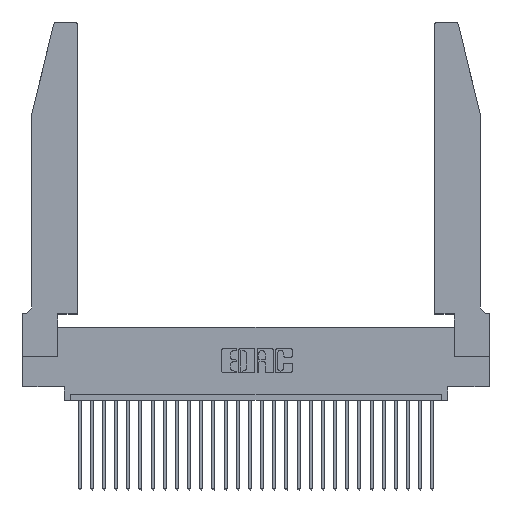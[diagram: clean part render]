
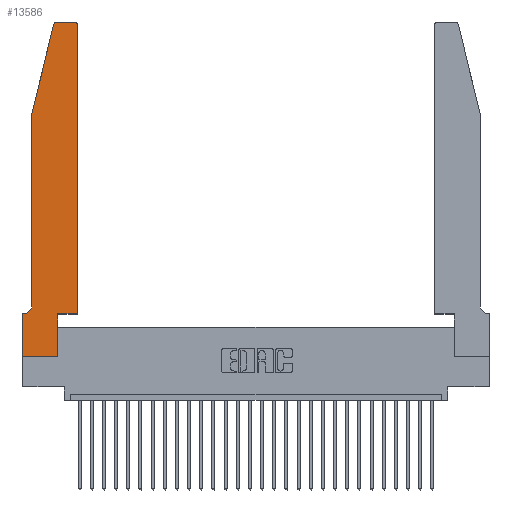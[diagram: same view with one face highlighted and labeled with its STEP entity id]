
A CAD part, top view. The second image highlights one B-rep face of the part: STEP entity #13586.
In plain terms, the highlighted planar face has unit normal (0, 0, 1).
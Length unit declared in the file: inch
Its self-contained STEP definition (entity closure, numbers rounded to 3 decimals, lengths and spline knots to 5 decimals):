
#89 = EDGE_LOOP ( 'NONE', ( #27496, #6674, #12539, #21687, #1411, #23947, #21259, #15491, #24205, #21631, #15594, #18094 ) ) ;
#479 = CIRCLE ( 'NONE', #1460, 0.03 ) ;
#762 = CIRCLE ( 'NONE', #11678, 0.03 ) ;
#1195 = CARTESIAN_POINT ( 'NONE',  ( 0.0755, 0.35, 0.37 ) ) ;
#1411 = ORIENTED_EDGE ( 'NONE', *, *, #18898, .T. ) ;
#1460 = AXIS2_PLACEMENT_3D ( 'NONE', #28780, #13288, #13474 ) ;
#1652 = VECTOR ( 'NONE', #7320, 39.37008 ) ;
#1716 = LINE ( 'NONE', #27912, #24635 ) ;
#1842 = EDGE_CURVE ( 'NONE', #8224, #24900, #9375, .T. ) ;
#1950 = EDGE_CURVE ( 'NONE', #25447, #23600, #9041, .T. ) ;
#1975 = EDGE_CURVE ( 'NONE', #24900, #28702, #24199, .T. ) ;
#2297 = DIRECTION ( 'NONE',  ( 0., -1., 0. ) ) ;
#2299 = CARTESIAN_POINT ( 'NONE',  ( 0.4505, 0.35, 0.37 ) ) ;
#2586 = CARTESIAN_POINT ( 'NONE',  ( 0.4205, 2.72, 0.37 ) ) ;
#2910 = CARTESIAN_POINT ( 'NONE',  ( 0.4505, 0.35, 0.37 ) ) ;
#3009 = VECTOR ( 'NONE', #19005, 39.37008 ) ;
#3139 = CARTESIAN_POINT ( 'NONE',  ( 0., 0.35, 0.37 ) ) ;
#3147 = DIRECTION ( 'NONE',  ( 0., 1., 0. ) ) ;
#3541 = CARTESIAN_POINT ( 'NONE',  ( 0., 0.35, 0.37 ) ) ;
#3924 = CARTESIAN_POINT ( 'NONE',  ( 0., 0., 0.37 ) ) ;
#5821 = CARTESIAN_POINT ( 'NONE',  ( 0.2865, 0.35, 0.37 ) ) ;
#5975 = CARTESIAN_POINT ( 'NONE',  ( 0.4505, 2.72, 0.37 ) ) ;
#6007 = VECTOR ( 'NONE', #9335, 39.37008 ) ;
#6084 = LINE ( 'NONE', #1195, #14186 ) ;
#6195 = DIRECTION ( 'NONE',  ( 1., 0., 0. ) ) ;
#6674 = ORIENTED_EDGE ( 'NONE', *, *, #12364, .T. ) ;
#7122 = AXIS2_PLACEMENT_3D ( 'NONE', #3139, #7982, #6195 ) ;
#7320 = DIRECTION ( 'NONE',  ( 0., -1., 0. ) ) ;
#7804 = CARTESIAN_POINT ( 'NONE',  ( 0.2605, 2.75, 0.37 ) ) ;
#7982 = DIRECTION ( 'NONE',  ( 0., 0., 1. ) ) ;
#8064 = EDGE_CURVE ( 'NONE', #21774, #8224, #6084, .T. ) ;
#8224 = VERTEX_POINT ( 'NONE', #3541 ) ;
#8480 = PLANE ( 'NONE',  #7122 ) ;
#9041 = LINE ( 'NONE', #27395, #9745 ) ;
#9335 = DIRECTION ( 'NONE',  ( 1., 0., 0. ) ) ;
#9375 = LINE ( 'NONE', #25190, #1652 ) ;
#9668 = DIRECTION ( 'NONE',  ( 1., 0., 0. ) ) ;
#9745 = VECTOR ( 'NONE', #2297, 39.37008 ) ;
#9904 = CARTESIAN_POINT ( 'NONE',  ( 0.0055, 0.35, 0.37 ) ) ;
#10312 = CARTESIAN_POINT ( 'NONE',  ( 0.25487, 2.72718, 0.37 ) ) ;
#10674 = FACE_OUTER_BOUND ( 'NONE', #89, .T. ) ;
#11245 = EDGE_CURVE ( 'NONE', #26189, #24770, #24901, .T. ) ;
#11678 = AXIS2_PLACEMENT_3D ( 'NONE', #2586, #13980, #9668 ) ;
#11720 = VERTEX_POINT ( 'NONE', #21074 ) ;
#11936 = DIRECTION ( 'NONE',  ( -1., 0., 0. ) ) ;
#12044 = CARTESIAN_POINT ( 'NONE',  ( 0.0055, 0.42, 0.37 ) ) ;
#12217 = VECTOR ( 'NONE', #22339, 39.37008 ) ;
#12364 = EDGE_CURVE ( 'NONE', #28287, #26040, #479, .T. ) ;
#12539 = ORIENTED_EDGE ( 'NONE', *, *, #19051, .T. ) ;
#13288 = DIRECTION ( 'NONE',  ( 0., 0., 1. ) ) ;
#13474 = DIRECTION ( 'NONE',  ( 1., 0., 0. ) ) ;
#13586 = ADVANCED_FACE ( 'NONE', ( #10674 ), #8480, .T. ) ;
#13980 = DIRECTION ( 'NONE',  ( 0., 0., 1. ) ) ;
#14186 = VECTOR ( 'NONE', #23722, 39.37008 ) ;
#14214 = AXIS2_PLACEMENT_3D ( 'NONE', #12044, #18595, #11936 ) ;
#14580 = DIRECTION ( 'NONE',  ( -0.239, -0.971, 0. ) ) ;
#14639 = EDGE_CURVE ( 'NONE', #24770, #25702, #762, .T. ) ;
#15466 = CIRCLE ( 'NONE', #14214, 0.07 ) ;
#15491 = ORIENTED_EDGE ( 'NONE', *, *, #1975, .T. ) ;
#15594 = ORIENTED_EDGE ( 'NONE', *, *, #11245, .T. ) ;
#16029 = CARTESIAN_POINT ( 'NONE',  ( 0.4205, 2.75, 0.37 ) ) ;
#18094 = ORIENTED_EDGE ( 'NONE', *, *, #14639, .T. ) ;
#18595 = DIRECTION ( 'NONE',  ( 0., 0., -1. ) ) ;
#18861 = VECTOR ( 'NONE', #3147, 39.37008 ) ;
#18898 = EDGE_CURVE ( 'NONE', #23600, #21774, #15466, .T. ) ;
#19005 = DIRECTION ( 'NONE',  ( -1., 0., 0. ) ) ;
#19051 = EDGE_CURVE ( 'NONE', #26040, #25447, #1716, .T. ) ;
#19381 = CARTESIAN_POINT ( 'NONE',  ( 0.0755, 2., 0.37 ) ) ;
#20538 = EDGE_CURVE ( 'NONE', #25702, #28287, #28339, .T. ) ;
#21074 = CARTESIAN_POINT ( 'NONE',  ( 0.2865, 0.35, 0.37 ) ) ;
#21135 = CARTESIAN_POINT ( 'NONE',  ( 0.2865, 0., 0.37 ) ) ;
#21259 = ORIENTED_EDGE ( 'NONE', *, *, #1842, .T. ) ;
#21631 = ORIENTED_EDGE ( 'NONE', *, *, #25914, .T. ) ;
#21687 = ORIENTED_EDGE ( 'NONE', *, *, #1950, .T. ) ;
#21774 = VERTEX_POINT ( 'NONE', #9904 ) ;
#22339 = DIRECTION ( 'NONE',  ( 1., 0., 0. ) ) ;
#22539 = EDGE_CURVE ( 'NONE', #28702, #11720, #27310, .T. ) ;
#22925 = LINE ( 'NONE', #2910, #6007 ) ;
#23600 = VERTEX_POINT ( 'NONE', #27965 ) ;
#23722 = DIRECTION ( 'NONE',  ( -1., 0., 0. ) ) ;
#23947 = ORIENTED_EDGE ( 'NONE', *, *, #8064, .T. ) ;
#24037 = CARTESIAN_POINT ( 'NONE',  ( 0.284, 2.75, 0.37 ) ) ;
#24199 = LINE ( 'NONE', #26215, #12217 ) ;
#24205 = ORIENTED_EDGE ( 'NONE', *, *, #22539, .T. ) ;
#24635 = VECTOR ( 'NONE', #14580, 39.37008 ) ;
#24770 = VERTEX_POINT ( 'NONE', #5975 ) ;
#24900 = VERTEX_POINT ( 'NONE', #3924 ) ;
#24901 = LINE ( 'NONE', #2299, #18861 ) ;
#25190 = CARTESIAN_POINT ( 'NONE',  ( 0., 0., 0.37 ) ) ;
#25447 = VERTEX_POINT ( 'NONE', #19381 ) ;
#25702 = VERTEX_POINT ( 'NONE', #16029 ) ;
#25914 = EDGE_CURVE ( 'NONE', #11720, #26189, #22925, .T. ) ;
#26040 = VERTEX_POINT ( 'NONE', #10312 ) ;
#26189 = VERTEX_POINT ( 'NONE', #26926 ) ;
#26215 = CARTESIAN_POINT ( 'NONE',  ( 0., 0., 0.37 ) ) ;
#26926 = CARTESIAN_POINT ( 'NONE',  ( 0.4505, 0.35, 0.37 ) ) ;
#27310 = LINE ( 'NONE', #5821, #29017 ) ;
#27395 = CARTESIAN_POINT ( 'NONE',  ( 0.0755, 2., 0.37 ) ) ;
#27496 = ORIENTED_EDGE ( 'NONE', *, *, #20538, .T. ) ;
#27912 = CARTESIAN_POINT ( 'NONE',  ( 0.0755, 2., 0.37 ) ) ;
#27965 = CARTESIAN_POINT ( 'NONE',  ( 0.0755, 0.42, 0.37 ) ) ;
#28287 = VERTEX_POINT ( 'NONE', #24037 ) ;
#28313 = DIRECTION ( 'NONE',  ( 0., 1., 0. ) ) ;
#28339 = LINE ( 'NONE', #7804, #3009 ) ;
#28702 = VERTEX_POINT ( 'NONE', #21135 ) ;
#28780 = CARTESIAN_POINT ( 'NONE',  ( 0.284, 2.72, 0.37 ) ) ;
#29017 = VECTOR ( 'NONE', #28313, 39.37008 ) ;
